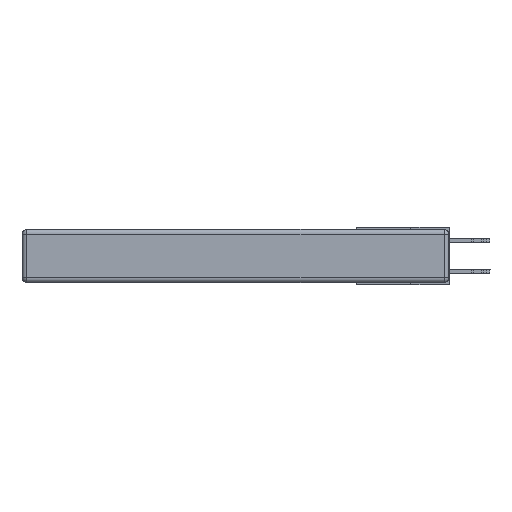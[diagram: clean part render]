
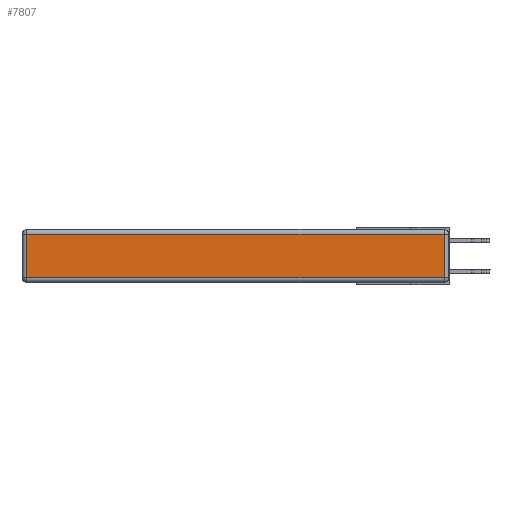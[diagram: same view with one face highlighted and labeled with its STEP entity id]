
A CAD part, left-side view. The second image highlights one B-rep face of the part: STEP entity #7807.
In plain terms, the highlighted planar face has unit normal (-1, 0, 0).
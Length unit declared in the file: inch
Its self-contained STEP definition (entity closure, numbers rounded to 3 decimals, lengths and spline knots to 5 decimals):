
#268 = EDGE_CURVE ( 'NONE', #12077, #1197, #23245, .T. ) ;
#886 = VERTEX_POINT ( 'NONE', #20999 ) ;
#1197 = VERTEX_POINT ( 'NONE', #11147 ) ;
#1205 = AXIS2_PLACEMENT_3D ( 'NONE', #28434, #26116, #12212 ) ;
#2618 = EDGE_CURVE ( 'NONE', #1197, #11018, #22368, .T. ) ;
#5187 = LINE ( 'NONE', #15918, #21638 ) ;
#6387 = ORIENTED_EDGE ( 'NONE', *, *, #12133, .T. ) ;
#6951 = DIRECTION ( 'NONE',  ( 0., -1., 0. ) ) ;
#7320 = CARTESIAN_POINT ( 'NONE',  ( 0., 2.72, -0.03 ) ) ;
#7807 = ADVANCED_FACE ( 'NONE', ( #18709 ), #12011, .T. ) ;
#7821 = DIRECTION ( 'NONE',  ( 0., 1., 0. ) ) ;
#9234 = CARTESIAN_POINT ( 'NONE',  ( 0., 2.72, -0.343 ) ) ;
#10132 = VECTOR ( 'NONE', #25488, 39.37008 ) ;
#11018 = VERTEX_POINT ( 'NONE', #18778 ) ;
#11147 = CARTESIAN_POINT ( 'NONE',  ( 0., 2.72, -0.313 ) ) ;
#12011 = PLANE ( 'NONE',  #1205 ) ;
#12077 = VERTEX_POINT ( 'NONE', #7320 ) ;
#12133 = EDGE_CURVE ( 'NONE', #886, #12077, #23700, .T. ) ;
#12212 = DIRECTION ( 'NONE',  ( 0., 0., 1. ) ) ;
#12903 = VECTOR ( 'NONE', #6951, 39.37008 ) ;
#14965 = VECTOR ( 'NONE', #7821, 39.37008 ) ;
#15918 = CARTESIAN_POINT ( 'NONE',  ( 0., 0.03, -0.343 ) ) ;
#16705 = DIRECTION ( 'NONE',  ( 0., 0., 1. ) ) ;
#18709 = FACE_OUTER_BOUND ( 'NONE', #29758, .T. ) ;
#18778 = CARTESIAN_POINT ( 'NONE',  ( 0., 0.03, -0.313 ) ) ;
#19799 = CARTESIAN_POINT ( 'NONE',  ( 0., 2.75, -0.03 ) ) ;
#20696 = CARTESIAN_POINT ( 'NONE',  ( 0., 0., -0.313 ) ) ;
#20999 = CARTESIAN_POINT ( 'NONE',  ( 0., 0.03, -0.03 ) ) ;
#21435 = ORIENTED_EDGE ( 'NONE', *, *, #268, .T. ) ;
#21638 = VECTOR ( 'NONE', #16705, 39.37008 ) ;
#22368 = LINE ( 'NONE', #20696, #12903 ) ;
#22470 = EDGE_CURVE ( 'NONE', #11018, #886, #5187, .T. ) ;
#23017 = ORIENTED_EDGE ( 'NONE', *, *, #2618, .T. ) ;
#23245 = LINE ( 'NONE', #9234, #10132 ) ;
#23700 = LINE ( 'NONE', #19799, #14965 ) ;
#25488 = DIRECTION ( 'NONE',  ( 0., 0., -1. ) ) ;
#26116 = DIRECTION ( 'NONE',  ( -1., 0., 0. ) ) ;
#28434 = CARTESIAN_POINT ( 'NONE',  ( 0., 0., -0.343 ) ) ;
#28524 = ORIENTED_EDGE ( 'NONE', *, *, #22470, .T. ) ;
#29758 = EDGE_LOOP ( 'NONE', ( #23017, #28524, #6387, #21435 ) ) ;
